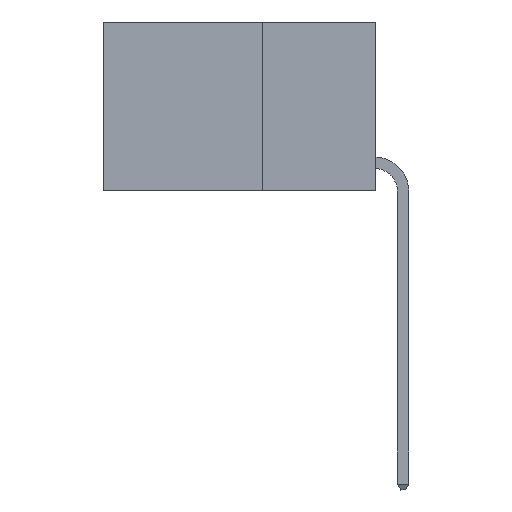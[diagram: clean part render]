
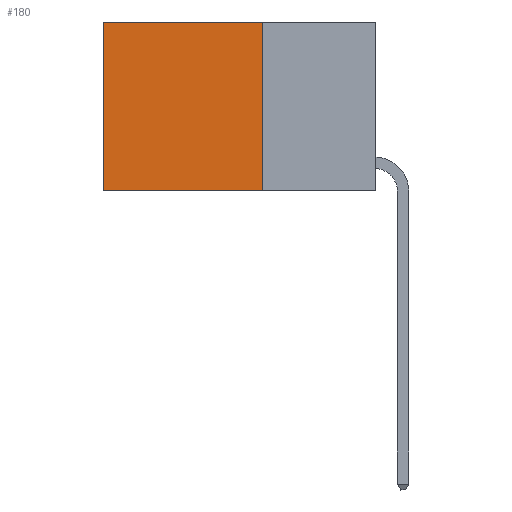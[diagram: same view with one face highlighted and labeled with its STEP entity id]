
A CAD part, left-side view. The second image highlights one B-rep face of the part: STEP entity #180.
In plain terms, the highlighted planar face has unit normal (-1, 0, 0).
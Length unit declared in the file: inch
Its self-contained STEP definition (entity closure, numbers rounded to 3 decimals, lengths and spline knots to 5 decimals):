
#180 = ADVANCED_FACE ( 'NONE', ( #6681 ), #14621, .F. ) ;
#958 = EDGE_CURVE ( 'NONE', #3263, #13628, #9292, .T. ) ;
#1400 = CARTESIAN_POINT ( 'NONE',  ( 0.2625, 0.25, 0. ) ) ;
#1522 = CARTESIAN_POINT ( 'NONE',  ( 0.2625, 0.25, 0. ) ) ;
#1703 = CARTESIAN_POINT ( 'NONE',  ( 0.2625, 0.6, 0. ) ) ;
#2039 = DIRECTION ( 'NONE',  ( 0., 1., 0. ) ) ;
#2190 = VECTOR ( 'NONE', #3110, 39.37008 ) ;
#2387 = VERTEX_POINT ( 'NONE', #5471 ) ;
#2782 = AXIS2_PLACEMENT_3D ( 'NONE', #1522, #2830, #15926 ) ;
#2830 = DIRECTION ( 'NONE',  ( 1., 0., 0. ) ) ;
#3110 = DIRECTION ( 'NONE',  ( 0., 1., 0. ) ) ;
#3263 = VERTEX_POINT ( 'NONE', #11900 ) ;
#4242 = VECTOR ( 'NONE', #14500, 39.37008 ) ;
#5392 = VECTOR ( 'NONE', #13563, 39.37008 ) ;
#5471 = CARTESIAN_POINT ( 'NONE',  ( 0.2625, 0.6, -0.37 ) ) ;
#6171 = CARTESIAN_POINT ( 'NONE',  ( 0.2625, 0.25, -0.37 ) ) ;
#6681 = FACE_OUTER_BOUND ( 'NONE', #10086, .T. ) ;
#9292 = LINE ( 'NONE', #1400, #4242 ) ;
#9515 = EDGE_CURVE ( 'NONE', #13707, #2387, #16061, .T. ) ;
#10067 = VECTOR ( 'NONE', #2039, 39.37008 ) ;
#10086 = EDGE_LOOP ( 'NONE', ( #10225, #14875, #16605, #11890 ) ) ;
#10225 = ORIENTED_EDGE ( 'NONE', *, *, #9515, .T. ) ;
#11113 = CARTESIAN_POINT ( 'NONE',  ( 0.2625, 0.25, 0. ) ) ;
#11890 = ORIENTED_EDGE ( 'NONE', *, *, #12289, .T. ) ;
#11900 = CARTESIAN_POINT ( 'NONE',  ( 0.2625, 0.25, 0. ) ) ;
#12284 = CARTESIAN_POINT ( 'NONE',  ( 0.2625, 0.6, 0. ) ) ;
#12289 = EDGE_CURVE ( 'NONE', #3263, #13707, #16343, .T. ) ;
#12344 = LINE ( 'NONE', #14997, #2190 ) ;
#13563 = DIRECTION ( 'NONE',  ( 0., 0., -1. ) ) ;
#13628 = VERTEX_POINT ( 'NONE', #6171 ) ;
#13707 = VERTEX_POINT ( 'NONE', #1703 ) ;
#14500 = DIRECTION ( 'NONE',  ( 0., 0., -1. ) ) ;
#14621 = PLANE ( 'NONE',  #2782 ) ;
#14875 = ORIENTED_EDGE ( 'NONE', *, *, #15189, .F. ) ;
#14997 = CARTESIAN_POINT ( 'NONE',  ( 0.2625, 0.25, -0.37 ) ) ;
#15189 = EDGE_CURVE ( 'NONE', #13628, #2387, #12344, .T. ) ;
#15926 = DIRECTION ( 'NONE',  ( 0., 0., -1. ) ) ;
#16061 = LINE ( 'NONE', #12284, #5392 ) ;
#16343 = LINE ( 'NONE', #11113, #10067 ) ;
#16605 = ORIENTED_EDGE ( 'NONE', *, *, #958, .F. ) ;
